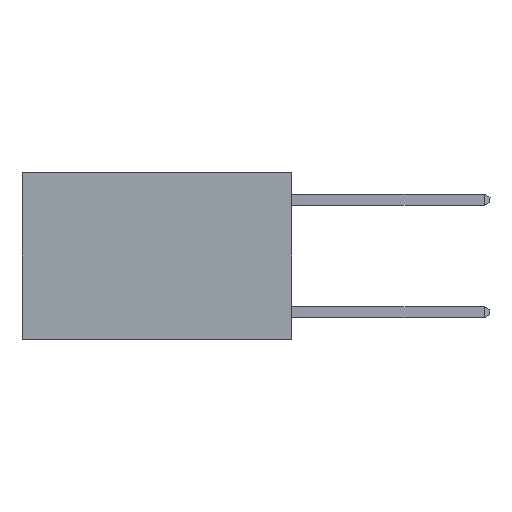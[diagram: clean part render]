
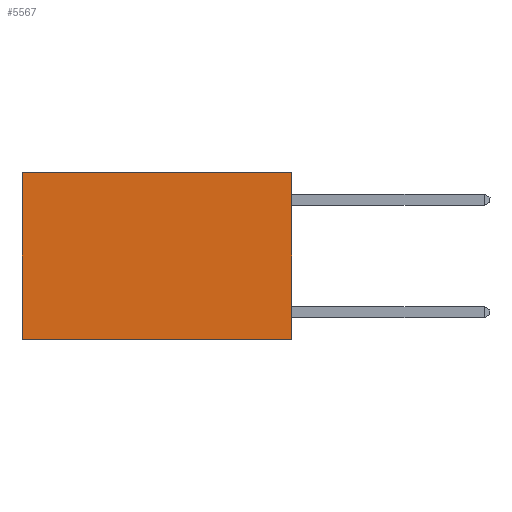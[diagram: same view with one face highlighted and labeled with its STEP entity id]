
A CAD part, left-side view. The second image highlights one B-rep face of the part: STEP entity #5567.
In plain terms, the highlighted planar face has unit normal (-1, 0, 0).
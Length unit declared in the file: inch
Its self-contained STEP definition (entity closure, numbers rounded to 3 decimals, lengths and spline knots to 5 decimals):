
#273 = LINE ( 'NONE', #9587, #8323 ) ;
#443 = CARTESIAN_POINT ( 'NONE',  ( 0.2625, 0.6, -0.37 ) ) ;
#695 = CARTESIAN_POINT ( 'NONE',  ( 0.2625, 0., 0. ) ) ;
#809 = ORIENTED_EDGE ( 'NONE', *, *, #3885, .F. ) ;
#861 = LINE ( 'NONE', #5205, #8408 ) ;
#871 = DIRECTION ( 'NONE',  ( 0., 1., 0. ) ) ;
#927 = CARTESIAN_POINT ( 'NONE',  ( 0.2625, 0., 0. ) ) ;
#1999 = VERTEX_POINT ( 'NONE', #443 ) ;
#2759 = VERTEX_POINT ( 'NONE', #695 ) ;
#3168 = ORIENTED_EDGE ( 'NONE', *, *, #3820, .T. ) ;
#3429 = DIRECTION ( 'NONE',  ( 1., 0., 0. ) ) ;
#3820 = EDGE_CURVE ( 'NONE', #2759, #4956, #7636, .T. ) ;
#3885 = EDGE_CURVE ( 'NONE', #2759, #4374, #6962, .T. ) ;
#4374 = VERTEX_POINT ( 'NONE', #4468 ) ;
#4468 = CARTESIAN_POINT ( 'NONE',  ( 0.2625, 0., -0.37 ) ) ;
#4741 = FACE_OUTER_BOUND ( 'NONE', #7693, .T. ) ;
#4843 = ORIENTED_EDGE ( 'NONE', *, *, #8132, .T. ) ;
#4956 = VERTEX_POINT ( 'NONE', #5123 ) ;
#5123 = CARTESIAN_POINT ( 'NONE',  ( 0.2625, 0.6, 0. ) ) ;
#5127 = ORIENTED_EDGE ( 'NONE', *, *, #9974, .F. ) ;
#5205 = CARTESIAN_POINT ( 'NONE',  ( 0.2625, 0., -0.37 ) ) ;
#5567 = ADVANCED_FACE ( 'NONE', ( #4741 ), #9483, .F. ) ;
#6226 = AXIS2_PLACEMENT_3D ( 'NONE', #7976, #3429, #8759 ) ;
#6359 = CARTESIAN_POINT ( 'NONE',  ( 0.2625, 0., 0. ) ) ;
#6962 = LINE ( 'NONE', #6359, #8735 ) ;
#7327 = DIRECTION ( 'NONE',  ( 0., 0., -1. ) ) ;
#7636 = LINE ( 'NONE', #927, #9432 ) ;
#7693 = EDGE_LOOP ( 'NONE', ( #4843, #5127, #809, #3168 ) ) ;
#7976 = CARTESIAN_POINT ( 'NONE',  ( 0.2625, 0., 0. ) ) ;
#8132 = EDGE_CURVE ( 'NONE', #4956, #1999, #273, .T. ) ;
#8186 = DIRECTION ( 'NONE',  ( 0., 1., 0. ) ) ;
#8323 = VECTOR ( 'NONE', #7327, 39.37008 ) ;
#8408 = VECTOR ( 'NONE', #8186, 39.37008 ) ;
#8487 = DIRECTION ( 'NONE',  ( 0., 0., -1. ) ) ;
#8735 = VECTOR ( 'NONE', #8487, 39.37008 ) ;
#8759 = DIRECTION ( 'NONE',  ( 0., 0., -1. ) ) ;
#9432 = VECTOR ( 'NONE', #871, 39.37008 ) ;
#9483 = PLANE ( 'NONE',  #6226 ) ;
#9587 = CARTESIAN_POINT ( 'NONE',  ( 0.2625, 0.6, 0. ) ) ;
#9974 = EDGE_CURVE ( 'NONE', #4374, #1999, #861, .T. ) ;
